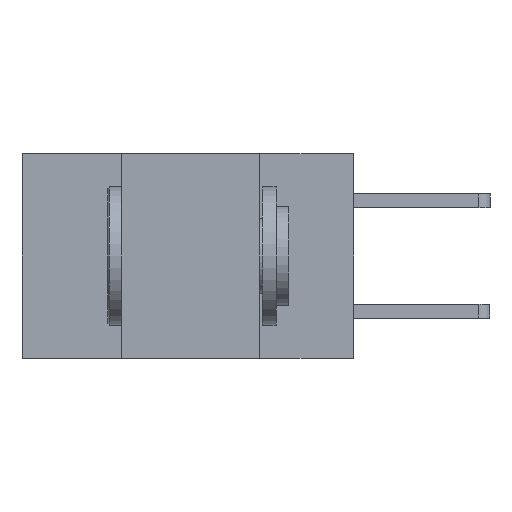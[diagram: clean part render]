
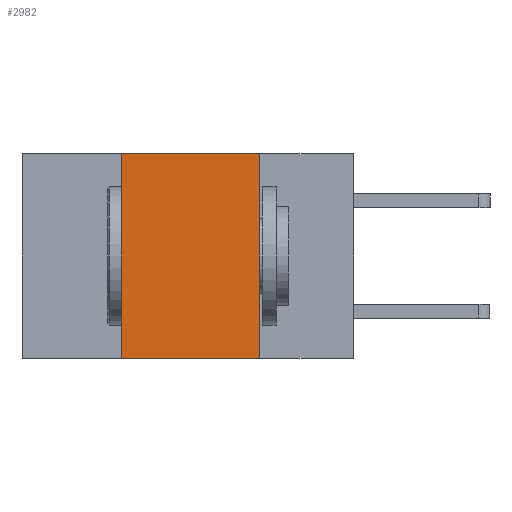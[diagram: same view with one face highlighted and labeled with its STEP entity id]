
A CAD part, left-side view. The second image highlights one B-rep face of the part: STEP entity #2982.
In plain terms, the highlighted planar face has unit normal (-1, 0, 0).
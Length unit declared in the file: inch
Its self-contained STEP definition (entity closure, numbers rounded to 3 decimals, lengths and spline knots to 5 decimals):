
#192 = ORIENTED_EDGE ( 'NONE', *, *, #908, .T. ) ;
#908 = EDGE_CURVE ( 'NONE', #8289, #5048, #5670, .T. ) ;
#2035 = CARTESIAN_POINT ( 'NONE',  ( 0., 0.17, 0. ) ) ;
#2149 = LINE ( 'NONE', #2035, #8844 ) ;
#2350 = FACE_OUTER_BOUND ( 'NONE', #7309, .T. ) ;
#2396 = CARTESIAN_POINT ( 'NONE',  ( 0., 0.6, 0. ) ) ;
#2982 = ADVANCED_FACE ( 'NONE', ( #2350 ), #4974, .F. ) ;
#3158 = DIRECTION ( 'NONE',  ( 1., 0., 0. ) ) ;
#3238 = CARTESIAN_POINT ( 'NONE',  ( 0., 0.42, 0. ) ) ;
#3477 = VECTOR ( 'NONE', #5008, 39.37008 ) ;
#3605 = CARTESIAN_POINT ( 'NONE',  ( 0., 0.17, 0. ) ) ;
#3632 = AXIS2_PLACEMENT_3D ( 'NONE', #2396, #3158, #4910 ) ;
#3872 = VECTOR ( 'NONE', #5100, 39.37008 ) ;
#4862 = EDGE_CURVE ( 'NONE', #10584, #5048, #2149, .T. ) ;
#4910 = DIRECTION ( 'NONE',  ( 0., 0., -1. ) ) ;
#4974 = PLANE ( 'NONE',  #3632 ) ;
#5008 = DIRECTION ( 'NONE',  ( 0., -1., 0. ) ) ;
#5048 = VERTEX_POINT ( 'NONE', #8117 ) ;
#5100 = DIRECTION ( 'NONE',  ( 0., 0., 1. ) ) ;
#5174 = LINE ( 'NONE', #9544, #3477 ) ;
#5436 = ORIENTED_EDGE ( 'NONE', *, *, #10839, .F. ) ;
#5667 = CARTESIAN_POINT ( 'NONE',  ( 0., 0.42, -0.37 ) ) ;
#5670 = LINE ( 'NONE', #9227, #7184 ) ;
#5983 = LINE ( 'NONE', #3238, #3872 ) ;
#7184 = VECTOR ( 'NONE', #7669, 39.37008 ) ;
#7309 = EDGE_LOOP ( 'NONE', ( #10418, #8418, #5436, #192 ) ) ;
#7669 = DIRECTION ( 'NONE',  ( 0., -1., 0. ) ) ;
#8117 = CARTESIAN_POINT ( 'NONE',  ( 0., 0.17, -0.37 ) ) ;
#8289 = VERTEX_POINT ( 'NONE', #5667 ) ;
#8418 = ORIENTED_EDGE ( 'NONE', *, *, #10225, .F. ) ;
#8640 = VERTEX_POINT ( 'NONE', #10058 ) ;
#8844 = VECTOR ( 'NONE', #9269, 39.37008 ) ;
#9227 = CARTESIAN_POINT ( 'NONE',  ( 0., 0.6, -0.37 ) ) ;
#9269 = DIRECTION ( 'NONE',  ( 0., 0., -1. ) ) ;
#9544 = CARTESIAN_POINT ( 'NONE',  ( 0., 0.6, 0. ) ) ;
#10058 = CARTESIAN_POINT ( 'NONE',  ( 0., 0.42, 0. ) ) ;
#10225 = EDGE_CURVE ( 'NONE', #8640, #10584, #5174, .T. ) ;
#10418 = ORIENTED_EDGE ( 'NONE', *, *, #4862, .F. ) ;
#10584 = VERTEX_POINT ( 'NONE', #3605 ) ;
#10839 = EDGE_CURVE ( 'NONE', #8289, #8640, #5983, .T. ) ;
